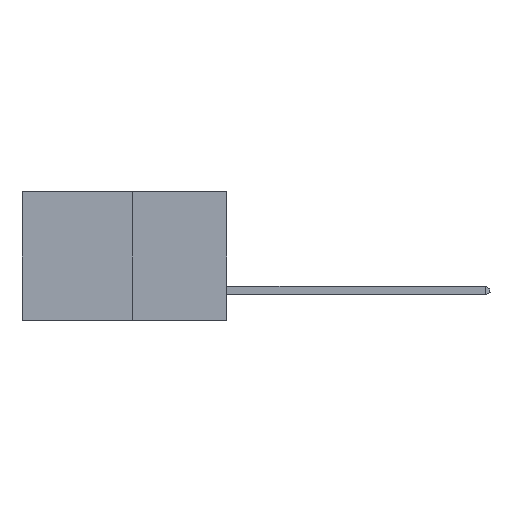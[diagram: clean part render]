
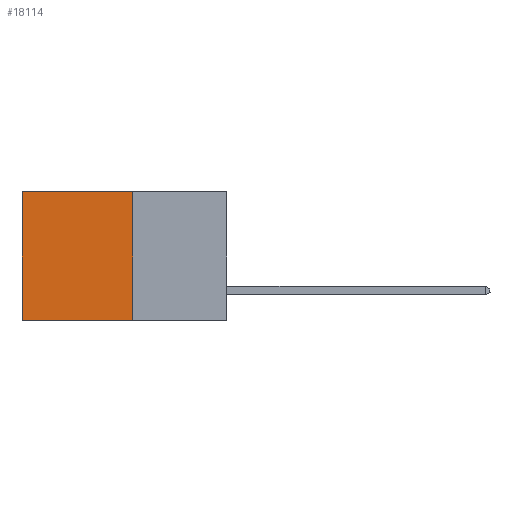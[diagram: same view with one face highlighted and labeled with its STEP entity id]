
A CAD part, left-side view. The second image highlights one B-rep face of the part: STEP entity #18114.
In plain terms, the highlighted planar face has unit normal (-1, 0, 0).
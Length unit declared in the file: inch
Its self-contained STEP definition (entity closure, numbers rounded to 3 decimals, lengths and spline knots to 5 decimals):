
#693 = LINE ( 'NONE', #11961, #9116 ) ;
#1024 = ORIENTED_EDGE ( 'NONE', *, *, #21077, .F. ) ;
#1049 = VECTOR ( 'NONE', #9786, 39.37008 ) ;
#1147 = FACE_OUTER_BOUND ( 'NONE', #14373, .T. ) ;
#1461 = CARTESIAN_POINT ( 'NONE',  ( 0.277, 0.27, -0.37 ) ) ;
#1568 = LINE ( 'NONE', #14922, #1049 ) ;
#2114 = ORIENTED_EDGE ( 'NONE', *, *, #12266, .F. ) ;
#3115 = LINE ( 'NONE', #7405, #10994 ) ;
#3413 = VERTEX_POINT ( 'NONE', #1461 ) ;
#4543 = VERTEX_POINT ( 'NONE', #7744 ) ;
#4562 = DIRECTION ( 'NONE',  ( 0., 0., -1. ) ) ;
#6041 = ORIENTED_EDGE ( 'NONE', *, *, #15132, .T. ) ;
#7405 = CARTESIAN_POINT ( 'NONE',  ( 0.277, 0.27, -0.37 ) ) ;
#7744 = CARTESIAN_POINT ( 'NONE',  ( 0.277, 0.59, 0. ) ) ;
#7861 = CARTESIAN_POINT ( 'NONE',  ( 0.277, 0.27, -0.37 ) ) ;
#8603 = EDGE_CURVE ( 'NONE', #15812, #4543, #693, .T. ) ;
#9116 = VECTOR ( 'NONE', #13678, 39.37008 ) ;
#9729 = AXIS2_PLACEMENT_3D ( 'NONE', #7861, #14691, #4562 ) ;
#9786 = DIRECTION ( 'NONE',  ( 0., 1., 0. ) ) ;
#10994 = VECTOR ( 'NONE', #15828, 39.37008 ) ;
#11116 = DIRECTION ( 'NONE',  ( 0., 0., -1. ) ) ;
#11961 = CARTESIAN_POINT ( 'NONE',  ( 0.277, 0.27, 0. ) ) ;
#12266 = EDGE_CURVE ( 'NONE', #3413, #20223, #1568, .T. ) ;
#12982 = PLANE ( 'NONE',  #9729 ) ;
#13085 = VECTOR ( 'NONE', #11116, 39.37008 ) ;
#13626 = LINE ( 'NONE', #16234, #13085 ) ;
#13678 = DIRECTION ( 'NONE',  ( 0., 1., 0. ) ) ;
#14373 = EDGE_LOOP ( 'NONE', ( #6041, #2114, #1024, #15889 ) ) ;
#14691 = DIRECTION ( 'NONE',  ( 1., 0., 0. ) ) ;
#14922 = CARTESIAN_POINT ( 'NONE',  ( 0.277, 0.27, -0.37 ) ) ;
#15132 = EDGE_CURVE ( 'NONE', #4543, #20223, #13626, .T. ) ;
#15812 = VERTEX_POINT ( 'NONE', #21327 ) ;
#15828 = DIRECTION ( 'NONE',  ( 0., 0., -1. ) ) ;
#15889 = ORIENTED_EDGE ( 'NONE', *, *, #8603, .T. ) ;
#16234 = CARTESIAN_POINT ( 'NONE',  ( 0.277, 0.59, -0.37 ) ) ;
#16792 = CARTESIAN_POINT ( 'NONE',  ( 0.277, 0.59, -0.37 ) ) ;
#18114 = ADVANCED_FACE ( 'NONE', ( #1147 ), #12982, .F. ) ;
#20223 = VERTEX_POINT ( 'NONE', #16792 ) ;
#21077 = EDGE_CURVE ( 'NONE', #15812, #3413, #3115, .T. ) ;
#21327 = CARTESIAN_POINT ( 'NONE',  ( 0.277, 0.27, 0. ) ) ;
